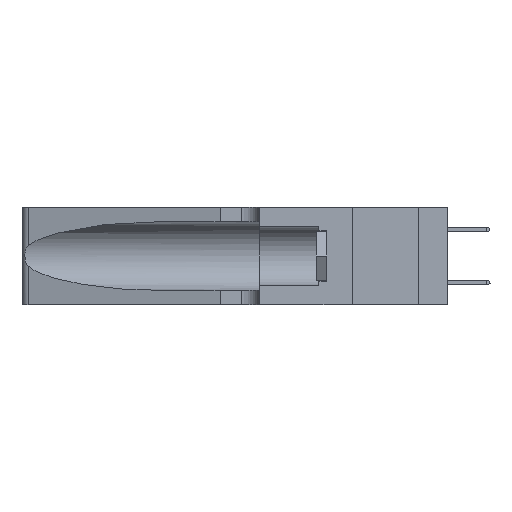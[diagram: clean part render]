
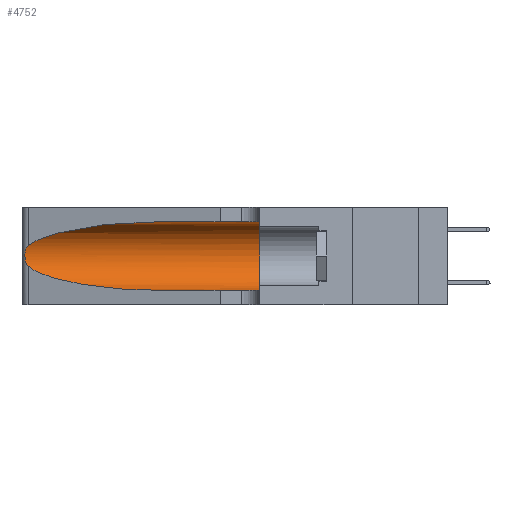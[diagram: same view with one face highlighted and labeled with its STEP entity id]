
A CAD part, left-side view. The second image highlights one B-rep face of the part: STEP entity #4752.
In plain terms, the highlighted cylindrical face has radius 3.308 mm (diameter 6.617 mm), a partial arc.
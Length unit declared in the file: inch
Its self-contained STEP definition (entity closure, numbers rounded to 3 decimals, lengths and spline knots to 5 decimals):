
#300 = DIRECTION ( 'NONE',  ( 0., -1., 0. ) ) ;
#354 =( BOUNDED_CURVE ( )  B_SPLINE_CURVE ( 3, ( #19994, #24361, #26513, #13574 ),
 .UNSPECIFIED., .F., .T. ) 
 B_SPLINE_CURVE_WITH_KNOTS ( ( 4, 4 ),
 ( 3.44316, 4.71239 ),
 .UNSPECIFIED. ) 
 CURVE ( )  GEOMETRIC_REPRESENTATION_ITEM ( )  RATIONAL_B_SPLINE_CURVE ( ( 1., 0.87, 0.87, 1. ) ) 
 REPRESENTATION_ITEM ( '' )  );
#436 = ORIENTED_EDGE ( 'NONE', *, *, #24076, .T. ) ;
#1085 = B_SPLINE_CURVE_WITH_KNOTS ( 'NONE', 3,
 ( #10861, #22217, #23668, #22714, #7946, #23408, #24892, #10939, #11310, #7924, #7734, #5033, #24089, #15258 ),
 .UNSPECIFIED., .F., .F.,
 ( 4, 2, 2, 2, 2, 2, 4 ),
 ( 0., 0.00027, 0.00053, 0.00107, 0.0016, 0.00187, 0.00214 ),
 .UNSPECIFIED. ) ;
#1265 = CARTESIAN_POINT ( 'NONE',  ( 0.1305, 1.61858, 0.185 ) ) ;
#1375 = EDGE_CURVE ( 'NONE', #22252, #21436, #1085, .T. ) ;
#1427 = VECTOR ( 'NONE', #27181, 39.37008 ) ;
#1716 = AXIS2_PLACEMENT_3D ( 'NONE', #1265, #23076, #5710 ) ;
#3171 = CARTESIAN_POINT ( 'NONE',  ( 0.1305, 0.35, 0.185 ) ) ;
#3370 = CARTESIAN_POINT ( 'NONE',  ( 0.25487, 1.22718, 0.22369 ) ) ;
#3910 = EDGE_CURVE ( 'NONE', #21436, #21894, #354, .T. ) ;
#4053 = EDGE_CURVE ( 'NONE', #9269, #24882, #16511, .T. ) ;
#4752 = ADVANCED_FACE ( 'NONE', ( #10721 ), #21582, .F. ) ;
#5033 = CARTESIAN_POINT ( 'NONE',  ( 0.25639, 1.23186, 0.15144 ) ) ;
#5322 = EDGE_CURVE ( 'NONE', #21894, #24882, #24607, .T. ) ;
#5356 = DIRECTION ( 'NONE',  ( 0., 0., 1. ) ) ;
#5710 = DIRECTION ( 'NONE',  ( 0., 0., -1. ) ) ;
#6914 = CARTESIAN_POINT ( 'NONE',  ( 0.1305, 0.72297, 0.05475 ) ) ;
#7617 = CARTESIAN_POINT ( 'NONE',  ( 0.25487, 1.22718, 0.14631 ) ) ;
#7734 = CARTESIAN_POINT ( 'NONE',  ( 0.25789, 1.23486, 0.15765 ) ) ;
#7793 = CARTESIAN_POINT ( 'NONE',  ( 0.1305, 1.61858, 0.05475 ) ) ;
#7924 = CARTESIAN_POINT ( 'NONE',  ( 0.25856, 1.23593, 0.16098 ) ) ;
#7946 = CARTESIAN_POINT ( 'NONE',  ( 0.25854, 1.2359, 0.20912 ) ) ;
#9269 = VERTEX_POINT ( 'NONE', #15491 ) ;
#9689 = EDGE_LOOP ( 'NONE', ( #436, #20564, #14170, #24828, #20397, #17368 ) ) ;
#9843 = CARTESIAN_POINT ( 'NONE',  ( 0.1305, 0.72297, 0.31525 ) ) ;
#10721 = FACE_OUTER_BOUND ( 'NONE', #9689, .T. ) ;
#10861 = CARTESIAN_POINT ( 'NONE',  ( 0.25487, 1.22718, 0.22369 ) ) ;
#10939 = CARTESIAN_POINT ( 'NONE',  ( 0.26075, 1.23896, 0.178 ) ) ;
#11310 = CARTESIAN_POINT ( 'NONE',  ( 0.26017, 1.23833, 0.17102 ) ) ;
#13574 = CARTESIAN_POINT ( 'NONE',  ( 0.1305, 0.72297, 0.05475 ) ) ;
#14170 = ORIENTED_EDGE ( 'NONE', *, *, #3910, .T. ) ;
#14655 = CARTESIAN_POINT ( 'NONE',  ( 0.1305, 0.35, 0.05475 ) ) ;
#15258 = CARTESIAN_POINT ( 'NONE',  ( 0.25487, 1.22718, 0.14631 ) ) ;
#15491 = CARTESIAN_POINT ( 'NONE',  ( 0.1305, 0.35, 0.31525 ) ) ;
#16425 = CARTESIAN_POINT ( 'NONE',  ( 0.2373, 1.15595, 0.28018 ) ) ;
#16511 = CIRCLE ( 'NONE', #20861, 0.13025 ) ;
#17368 = ORIENTED_EDGE ( 'NONE', *, *, #26399, .F. ) ;
#18307 = VECTOR ( 'NONE', #300, 39.37008 ) ;
#18394 = DIRECTION ( 'NONE',  ( 0., 1., 0. ) ) ;
#19304 = VERTEX_POINT ( 'NONE', #20477 ) ;
#19994 = CARTESIAN_POINT ( 'NONE',  ( 0.25487, 1.22718, 0.14631 ) ) ;
#20397 = ORIENTED_EDGE ( 'NONE', *, *, #4053, .F. ) ;
#20477 = CARTESIAN_POINT ( 'NONE',  ( 0.1305, 0.72297, 0.31525 ) ) ;
#20564 = ORIENTED_EDGE ( 'NONE', *, *, #1375, .T. ) ;
#20861 = AXIS2_PLACEMENT_3D ( 'NONE', #3171, #18394, #5356 ) ;
#21436 = VERTEX_POINT ( 'NONE', #7617 ) ;
#21582 = CYLINDRICAL_SURFACE ( 'NONE', #1716, 0.13025 ) ;
#21894 = VERTEX_POINT ( 'NONE', #6914 ) ;
#22217 = CARTESIAN_POINT ( 'NONE',  ( 0.25555, 1.22994, 0.2215 ) ) ;
#22252 = VERTEX_POINT ( 'NONE', #23204 ) ;
#22714 = CARTESIAN_POINT ( 'NONE',  ( 0.25787, 1.23484, 0.2124 ) ) ;
#22846 = CARTESIAN_POINT ( 'NONE',  ( 0.18966, 0.96281, 0.31525 ) ) ;
#23076 = DIRECTION ( 'NONE',  ( 0., -1., 0. ) ) ;
#23204 = CARTESIAN_POINT ( 'NONE',  ( 0.25487, 1.22718, 0.22369 ) ) ;
#23241 =( BOUNDED_CURVE ( )  B_SPLINE_CURVE ( 3, ( #9843, #22846, #16425, #3370 ),
 .UNSPECIFIED., .F., .F. ) 
 B_SPLINE_CURVE_WITH_KNOTS ( ( 4, 4 ),
 ( 1.5708, 2.84003 ),
 .UNSPECIFIED. ) 
 CURVE ( )  GEOMETRIC_REPRESENTATION_ITEM ( )  RATIONAL_B_SPLINE_CURVE ( ( 1., 0.87, 0.87, 1. ) ) 
 REPRESENTATION_ITEM ( '' )  );
#23408 = CARTESIAN_POINT ( 'NONE',  ( 0.26018, 1.23835, 0.19895 ) ) ;
#23668 = CARTESIAN_POINT ( 'NONE',  ( 0.25639, 1.23184, 0.21858 ) ) ;
#24070 = LINE ( 'NONE', #24243, #18307 ) ;
#24076 = EDGE_CURVE ( 'NONE', #19304, #22252, #23241, .T. ) ;
#24089 = CARTESIAN_POINT ( 'NONE',  ( 0.25555, 1.22993, 0.14849 ) ) ;
#24243 = CARTESIAN_POINT ( 'NONE',  ( 0.1305, 1.61858, 0.31525 ) ) ;
#24361 = CARTESIAN_POINT ( 'NONE',  ( 0.2373, 1.15595, 0.08982 ) ) ;
#24607 = LINE ( 'NONE', #7793, #1427 ) ;
#24828 = ORIENTED_EDGE ( 'NONE', *, *, #5322, .T. ) ;
#24882 = VERTEX_POINT ( 'NONE', #14655 ) ;
#24892 = CARTESIAN_POINT ( 'NONE',  ( 0.26075, 1.23896, 0.19203 ) ) ;
#26399 = EDGE_CURVE ( 'NONE', #19304, #9269, #24070, .T. ) ;
#26513 = CARTESIAN_POINT ( 'NONE',  ( 0.18966, 0.96281, 0.05475 ) ) ;
#27181 = DIRECTION ( 'NONE',  ( 0., -1., 0. ) ) ;
